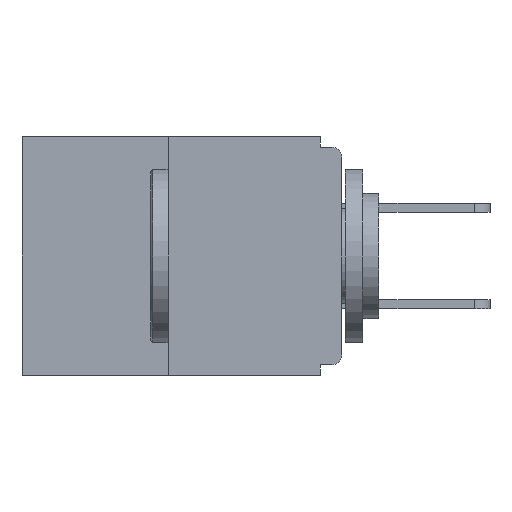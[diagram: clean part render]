
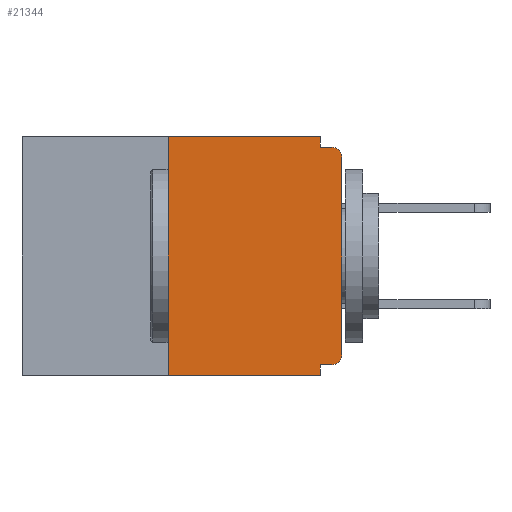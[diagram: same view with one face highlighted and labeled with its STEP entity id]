
A CAD part, left-side view. The second image highlights one B-rep face of the part: STEP entity #21344.
In plain terms, the highlighted planar face has unit normal (-1, 0, 0).
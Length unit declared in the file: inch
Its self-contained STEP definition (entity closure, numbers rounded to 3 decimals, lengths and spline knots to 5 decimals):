
#553 = CARTESIAN_POINT ( 'NONE',  ( 0., 0.25, 0. ) ) ;
#1059 = ORIENTED_EDGE ( 'NONE', *, *, #8421, .T. ) ;
#1271 = DIRECTION ( 'NONE',  ( 0., -1., 0. ) ) ;
#1406 = VERTEX_POINT ( 'NONE', #2321 ) ;
#2281 = LINE ( 'NONE', #16193, #14647 ) ;
#2321 = CARTESIAN_POINT ( 'NONE',  ( 0., 0.015, -0.328 ) ) ;
#2873 = CARTESIAN_POINT ( 'NONE',  ( 0., 0.031, 0. ) ) ;
#3807 = VERTEX_POINT ( 'NONE', #11914 ) ;
#4271 = DIRECTION ( 'NONE',  ( 1., 0., 0. ) ) ;
#4297 = DIRECTION ( 'NONE',  ( 0., 1., 0. ) ) ;
#4459 = AXIS2_PLACEMENT_3D ( 'NONE', #27133, #4271, #6527 ) ;
#4566 = LINE ( 'NONE', #553, #25010 ) ;
#4609 = ORIENTED_EDGE ( 'NONE', *, *, #7614, .F. ) ;
#5424 = EDGE_CURVE ( 'NONE', #26153, #3807, #4566, .T. ) ;
#5597 = CARTESIAN_POINT ( 'NONE',  ( 0., 0., -0.313 ) ) ;
#5779 = AXIS2_PLACEMENT_3D ( 'NONE', #21905, #29050, #24379 ) ;
#6360 = AXIS2_PLACEMENT_3D ( 'NONE', #28719, #19989, #19787 ) ;
#6408 = CARTESIAN_POINT ( 'NONE',  ( 0., 0.46, -0.343 ) ) ;
#6456 = VECTOR ( 'NONE', #1271, 39.37008 ) ;
#6500 = DIRECTION ( 'NONE',  ( 0., -1., 0. ) ) ;
#6527 = DIRECTION ( 'NONE',  ( 0., 0., -1. ) ) ;
#6710 = ORIENTED_EDGE ( 'NONE', *, *, #21639, .T. ) ;
#7174 = EDGE_CURVE ( 'NONE', #3807, #20538, #17670, .T. ) ;
#7304 = VECTOR ( 'NONE', #16697, 39.37008 ) ;
#7575 = ORIENTED_EDGE ( 'NONE', *, *, #7174, .F. ) ;
#7614 = EDGE_CURVE ( 'NONE', #20538, #27884, #10951, .T. ) ;
#8421 = EDGE_CURVE ( 'NONE', #19545, #8976, #13356, .T. ) ;
#8639 = ORIENTED_EDGE ( 'NONE', *, *, #5424, .F. ) ;
#8731 = CARTESIAN_POINT ( 'NONE',  ( 0., 0.031, 0. ) ) ;
#8920 = DIRECTION ( 'NONE',  ( 0., 0., -1. ) ) ;
#8976 = VERTEX_POINT ( 'NONE', #13391 ) ;
#9054 = LINE ( 'NONE', #19987, #11942 ) ;
#9486 = CARTESIAN_POINT ( 'NONE',  ( 0., 0.25, -0.343 ) ) ;
#10633 = CARTESIAN_POINT ( 'NONE',  ( 0., 0.015, -0.015 ) ) ;
#10951 = LINE ( 'NONE', #8731, #28555 ) ;
#11135 = VECTOR ( 'NONE', #6500, 39.37008 ) ;
#11914 = CARTESIAN_POINT ( 'NONE',  ( 0., 0.25, 0. ) ) ;
#11942 = VECTOR ( 'NONE', #4297, 39.37008 ) ;
#12453 = FACE_OUTER_BOUND ( 'NONE', #25361, .T. ) ;
#12473 = CARTESIAN_POINT ( 'NONE',  ( 0., 0.46, 0. ) ) ;
#12488 = ORIENTED_EDGE ( 'NONE', *, *, #21093, .F. ) ;
#13256 = PLANE ( 'NONE',  #4459 ) ;
#13356 = LINE ( 'NONE', #14799, #7304 ) ;
#13391 = CARTESIAN_POINT ( 'NONE',  ( 0., 0., -0.03 ) ) ;
#13519 = VERTEX_POINT ( 'NONE', #10633 ) ;
#14218 = DIRECTION ( 'NONE',  ( 0., 0., -1. ) ) ;
#14221 = LINE ( 'NONE', #28330, #6456 ) ;
#14647 = VECTOR ( 'NONE', #14218, 39.37008 ) ;
#14799 = CARTESIAN_POINT ( 'NONE',  ( 0., 0., 0. ) ) ;
#15085 = DIRECTION ( 'NONE',  ( 0., -1., 0. ) ) ;
#15251 = CIRCLE ( 'NONE', #5779, 0.015 ) ;
#16193 = CARTESIAN_POINT ( 'NONE',  ( 0., 0.031, -0.343 ) ) ;
#16697 = DIRECTION ( 'NONE',  ( 0., 0., 1. ) ) ;
#16923 = ORIENTED_EDGE ( 'NONE', *, *, #27839, .T. ) ;
#17670 = LINE ( 'NONE', #12473, #20464 ) ;
#18012 = CARTESIAN_POINT ( 'NONE',  ( 0., 0.031, -0.015 ) ) ;
#18057 = CARTESIAN_POINT ( 'NONE',  ( 0., 0.031, -0.343 ) ) ;
#18850 = DIRECTION ( 'NONE',  ( 0., 0., 1. ) ) ;
#19545 = VERTEX_POINT ( 'NONE', #5597 ) ;
#19787 = DIRECTION ( 'NONE',  ( 0., 0., -1. ) ) ;
#19987 = CARTESIAN_POINT ( 'NONE',  ( 0., 0., -0.328 ) ) ;
#19989 = DIRECTION ( 'NONE',  ( -1., 0., 0. ) ) ;
#20464 = VECTOR ( 'NONE', #15085, 39.37008 ) ;
#20538 = VERTEX_POINT ( 'NONE', #2873 ) ;
#21093 = EDGE_CURVE ( 'NONE', #27884, #13519, #14221, .T. ) ;
#21344 = ADVANCED_FACE ( 'NONE', ( #12453 ), #13256, .F. ) ;
#21639 = EDGE_CURVE ( 'NONE', #8976, #13519, #24744, .T. ) ;
#21866 = VERTEX_POINT ( 'NONE', #23362 ) ;
#21905 = CARTESIAN_POINT ( 'NONE',  ( 0., 0.015, -0.313 ) ) ;
#23362 = CARTESIAN_POINT ( 'NONE',  ( 0., 0.031, -0.328 ) ) ;
#23577 = EDGE_CURVE ( 'NONE', #1406, #21866, #9054, .T. ) ;
#24379 = DIRECTION ( 'NONE',  ( 0., 0., -1. ) ) ;
#24506 = LINE ( 'NONE', #6408, #11135 ) ;
#24744 = CIRCLE ( 'NONE', #6360, 0.015 ) ;
#25010 = VECTOR ( 'NONE', #18850, 39.37008 ) ;
#25352 = EDGE_CURVE ( 'NONE', #21866, #26562, #2281, .T. ) ;
#25361 = EDGE_LOOP ( 'NONE', ( #7575, #8639, #29088, #28758, #26714, #16923, #1059, #6710, #12488, #4609 ) ) ;
#26153 = VERTEX_POINT ( 'NONE', #9486 ) ;
#26516 = EDGE_CURVE ( 'NONE', #26153, #26562, #24506, .T. ) ;
#26562 = VERTEX_POINT ( 'NONE', #18057 ) ;
#26714 = ORIENTED_EDGE ( 'NONE', *, *, #23577, .F. ) ;
#27133 = CARTESIAN_POINT ( 'NONE',  ( 0., 0.46, 0. ) ) ;
#27839 = EDGE_CURVE ( 'NONE', #1406, #19545, #15251, .T. ) ;
#27884 = VERTEX_POINT ( 'NONE', #18012 ) ;
#28330 = CARTESIAN_POINT ( 'NONE',  ( 0., 0., -0.015 ) ) ;
#28555 = VECTOR ( 'NONE', #8920, 39.37008 ) ;
#28719 = CARTESIAN_POINT ( 'NONE',  ( 0., 0.015, -0.03 ) ) ;
#28758 = ORIENTED_EDGE ( 'NONE', *, *, #25352, .F. ) ;
#29050 = DIRECTION ( 'NONE',  ( -1., 0., 0. ) ) ;
#29088 = ORIENTED_EDGE ( 'NONE', *, *, #26516, .T. ) ;
